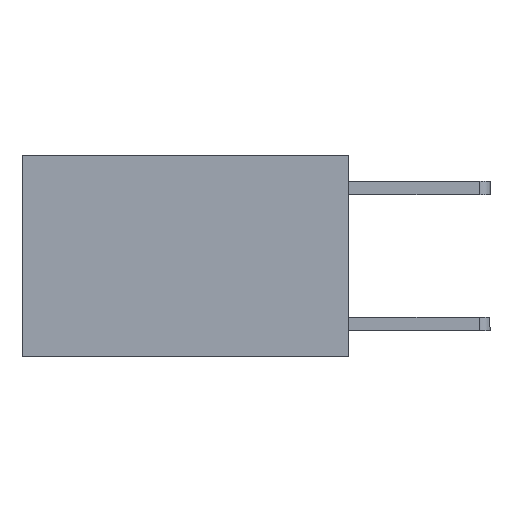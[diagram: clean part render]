
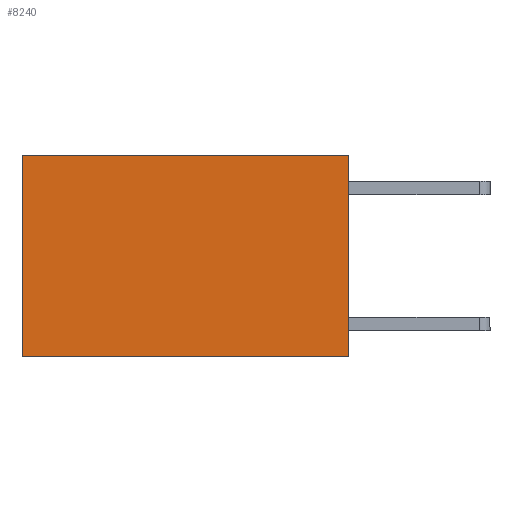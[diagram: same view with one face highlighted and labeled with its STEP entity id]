
A CAD part, left-side view. The second image highlights one B-rep face of the part: STEP entity #8240.
In plain terms, the highlighted planar face has unit normal (-1, 0, 0).
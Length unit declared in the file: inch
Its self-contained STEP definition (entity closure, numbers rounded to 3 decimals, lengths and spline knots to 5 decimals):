
#498 = DIRECTION ( 'NONE',  ( 0., 0., -1. ) ) ;
#528 = DIRECTION ( 'NONE',  ( 0., 0., -1. ) ) ;
#2154 = VECTOR ( 'NONE', #8295, 39.37008 ) ;
#2470 = DIRECTION ( 'NONE',  ( 0., 1., 0. ) ) ;
#2959 = VERTEX_POINT ( 'NONE', #3171 ) ;
#3057 = VECTOR ( 'NONE', #2470, 39.37008 ) ;
#3171 = CARTESIAN_POINT ( 'NONE',  ( 0.2625, 0., 0. ) ) ;
#3395 = EDGE_CURVE ( 'NONE', #8066, #8738, #9954, .T. ) ;
#3421 = CARTESIAN_POINT ( 'NONE',  ( 0.2625, 0., -0.37 ) ) ;
#3436 = VECTOR ( 'NONE', #498, 39.37008 ) ;
#3579 = VECTOR ( 'NONE', #7733, 39.37008 ) ;
#4310 = CARTESIAN_POINT ( 'NONE',  ( 0.2625, 0., 0. ) ) ;
#4890 = ORIENTED_EDGE ( 'NONE', *, *, #9058, .T. ) ;
#5230 = VERTEX_POINT ( 'NONE', #10587 ) ;
#5925 = LINE ( 'NONE', #4310, #3579 ) ;
#6285 = ORIENTED_EDGE ( 'NONE', *, *, #10625, .F. ) ;
#7387 = CARTESIAN_POINT ( 'NONE',  ( 0.2625, 0., 0. ) ) ;
#7469 = AXIS2_PLACEMENT_3D ( 'NONE', #8197, #9135, #528 ) ;
#7733 = DIRECTION ( 'NONE',  ( 0., 1., 0. ) ) ;
#8066 = VERTEX_POINT ( 'NONE', #9795 ) ;
#8190 = CARTESIAN_POINT ( 'NONE',  ( 0.2625, 0.6, 0. ) ) ;
#8197 = CARTESIAN_POINT ( 'NONE',  ( 0.2625, 0., 0. ) ) ;
#8240 = ADVANCED_FACE ( 'NONE', ( #9019 ), #9848, .F. ) ;
#8295 = DIRECTION ( 'NONE',  ( 0., 0., -1. ) ) ;
#8738 = VERTEX_POINT ( 'NONE', #9555 ) ;
#9019 = FACE_OUTER_BOUND ( 'NONE', #9737, .T. ) ;
#9058 = EDGE_CURVE ( 'NONE', #2959, #8066, #5925, .T. ) ;
#9064 = EDGE_CURVE ( 'NONE', #5230, #8738, #10105, .T. ) ;
#9135 = DIRECTION ( 'NONE',  ( 1., 0., 0. ) ) ;
#9555 = CARTESIAN_POINT ( 'NONE',  ( 0.2625, 0.6, -0.37 ) ) ;
#9737 = EDGE_LOOP ( 'NONE', ( #10334, #10604, #6285, #4890 ) ) ;
#9795 = CARTESIAN_POINT ( 'NONE',  ( 0.2625, 0.6, 0. ) ) ;
#9848 = PLANE ( 'NONE',  #7469 ) ;
#9954 = LINE ( 'NONE', #8190, #2154 ) ;
#10105 = LINE ( 'NONE', #3421, #3057 ) ;
#10334 = ORIENTED_EDGE ( 'NONE', *, *, #3395, .T. ) ;
#10587 = CARTESIAN_POINT ( 'NONE',  ( 0.2625, 0., -0.37 ) ) ;
#10604 = ORIENTED_EDGE ( 'NONE', *, *, #9064, .F. ) ;
#10625 = EDGE_CURVE ( 'NONE', #2959, #5230, #10822, .T. ) ;
#10822 = LINE ( 'NONE', #7387, #3436 ) ;
